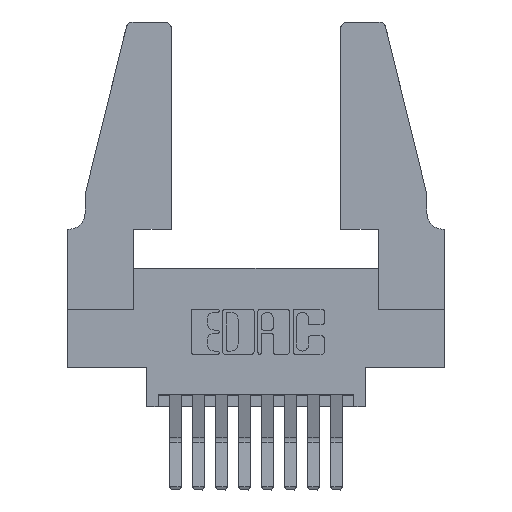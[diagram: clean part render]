
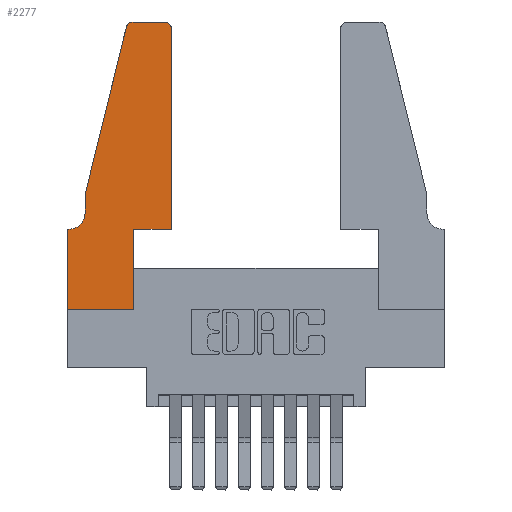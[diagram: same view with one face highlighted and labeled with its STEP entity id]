
A CAD part, top view. The second image highlights one B-rep face of the part: STEP entity #2277.
In plain terms, the highlighted planar face has unit normal (0, 0, 1).
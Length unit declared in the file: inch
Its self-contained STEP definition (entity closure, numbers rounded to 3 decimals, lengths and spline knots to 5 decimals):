
#139 = ORIENTED_EDGE ( 'NONE', *, *, #2441, .T. ) ;
#209 = CARTESIAN_POINT ( 'NONE',  ( 0.0755, 0.5, 0.37 ) ) ;
#359 = LINE ( 'NONE', #10617, #1563 ) ;
#665 = ORIENTED_EDGE ( 'NONE', *, *, #5520, .T. ) ;
#1165 = DIRECTION ( 'NONE',  ( 1., 0., 0. ) ) ;
#1204 = EDGE_CURVE ( 'NONE', #5422, #12656, #9728, .T. ) ;
#1392 = DIRECTION ( 'NONE',  ( -1., 0., 0. ) ) ;
#1563 = VECTOR ( 'NONE', #2473, 39.37008 ) ;
#1684 = DIRECTION ( 'NONE',  ( 0., -1., 0. ) ) ;
#1807 = VECTOR ( 'NONE', #3904, 39.37008 ) ;
#1826 = CARTESIAN_POINT ( 'NONE',  ( 0., 0., 0.37 ) ) ;
#2215 = VECTOR ( 'NONE', #1165, 39.37008 ) ;
#2277 = ADVANCED_FACE ( 'NONE', ( #2661 ), #8542, .T. ) ;
#2283 = VERTEX_POINT ( 'NONE', #11333 ) ;
#2441 = EDGE_CURVE ( 'NONE', #2283, #3994, #6580, .T. ) ;
#2448 = CIRCLE ( 'NONE', #3282, 0.03 ) ;
#2473 = DIRECTION ( 'NONE',  ( 0., 1., 0. ) ) ;
#2598 = CARTESIAN_POINT ( 'NONE',  ( 0.2865, 0.35, 0.37 ) ) ;
#2661 = FACE_OUTER_BOUND ( 'NONE', #2886, .T. ) ;
#2803 = LINE ( 'NONE', #9592, #13189 ) ;
#2817 = EDGE_CURVE ( 'NONE', #11545, #5595, #7525, .T. ) ;
#2837 = VERTEX_POINT ( 'NONE', #6873 ) ;
#2886 = EDGE_LOOP ( 'NONE', ( #139, #12139, #8908, #665, #12896, #9396, #6547, #11889, #8979, #6647, #8243, #10507 ) ) ;
#3049 = CARTESIAN_POINT ( 'NONE',  ( 0.0055, 0.35, 0.37 ) ) ;
#3071 = EDGE_CURVE ( 'NONE', #6088, #13042, #9677, .T. ) ;
#3072 = CARTESIAN_POINT ( 'NONE',  ( 0.4505, 0.35, 0.37 ) ) ;
#3123 = CARTESIAN_POINT ( 'NONE',  ( 0.4505, 0.35, 0.37 ) ) ;
#3135 = AXIS2_PLACEMENT_3D ( 'NONE', #8990, #8208, #11821 ) ;
#3225 = VERTEX_POINT ( 'NONE', #209 ) ;
#3266 = VECTOR ( 'NONE', #9991, 39.37008 ) ;
#3282 = AXIS2_PLACEMENT_3D ( 'NONE', #6283, #13174, #7293 ) ;
#3471 = EDGE_CURVE ( 'NONE', #12656, #11545, #2803, .T. ) ;
#3514 = VECTOR ( 'NONE', #6113, 39.37008 ) ;
#3708 = DIRECTION ( 'NONE',  ( 0., 0., -1. ) ) ;
#3747 = AXIS2_PLACEMENT_3D ( 'NONE', #7775, #3708, #11524 ) ;
#3904 = DIRECTION ( 'NONE',  ( 1., 0., 0. ) ) ;
#3994 = VERTEX_POINT ( 'NONE', #5449 ) ;
#4210 = EDGE_CURVE ( 'NONE', #3994, #2837, #5448, .T. ) ;
#4516 = VECTOR ( 'NONE', #7219, 39.37008 ) ;
#4773 = DIRECTION ( 'NONE',  ( 0., 0., 1. ) ) ;
#4895 = LINE ( 'NONE', #3123, #11602 ) ;
#5058 = LINE ( 'NONE', #5441, #2215 ) ;
#5085 = EDGE_CURVE ( 'NONE', #2837, #3225, #5741, .T. ) ;
#5121 = AXIS2_PLACEMENT_3D ( 'NONE', #10730, #4773, #11746 ) ;
#5422 = VERTEX_POINT ( 'NONE', #9725 ) ;
#5441 = CARTESIAN_POINT ( 'NONE',  ( 0., 0., 0.37 ) ) ;
#5448 = CIRCLE ( 'NONE', #5121, 0.03 ) ;
#5449 = CARTESIAN_POINT ( 'NONE',  ( 0.284, 1.25, 0.37 ) ) ;
#5520 = EDGE_CURVE ( 'NONE', #3225, #5422, #11314, .T. ) ;
#5595 = VERTEX_POINT ( 'NONE', #1826 ) ;
#5741 = LINE ( 'NONE', #8023, #3266 ) ;
#5845 = CARTESIAN_POINT ( 'NONE',  ( 0.4505, 0.35, 0.37 ) ) ;
#5930 = CARTESIAN_POINT ( 'NONE',  ( 0.4505, 1.22, 0.37 ) ) ;
#6038 = CARTESIAN_POINT ( 'NONE',  ( 0.2605, 1.25, 0.37 ) ) ;
#6088 = VERTEX_POINT ( 'NONE', #2598 ) ;
#6113 = DIRECTION ( 'NONE',  ( -1., 0., 0. ) ) ;
#6164 = VERTEX_POINT ( 'NONE', #5930 ) ;
#6283 = CARTESIAN_POINT ( 'NONE',  ( 0.4205, 1.22, 0.37 ) ) ;
#6367 = VERTEX_POINT ( 'NONE', #12958 ) ;
#6483 = EDGE_CURVE ( 'NONE', #13042, #6164, #4895, .T. ) ;
#6547 = ORIENTED_EDGE ( 'NONE', *, *, #2817, .T. ) ;
#6580 = LINE ( 'NONE', #6038, #3514 ) ;
#6608 = EDGE_CURVE ( 'NONE', #5595, #6367, #5058, .T. ) ;
#6647 = ORIENTED_EDGE ( 'NONE', *, *, #3071, .T. ) ;
#6873 = CARTESIAN_POINT ( 'NONE',  ( 0.25487, 1.22718, 0.37 ) ) ;
#7073 = CARTESIAN_POINT ( 'NONE',  ( 0., 0., 0.37 ) ) ;
#7219 = DIRECTION ( 'NONE',  ( 0., -1., 0. ) ) ;
#7293 = DIRECTION ( 'NONE',  ( 1., 0., 0. ) ) ;
#7525 = LINE ( 'NONE', #7073, #4516 ) ;
#7775 = CARTESIAN_POINT ( 'NONE',  ( 0.0055, 0.42, 0.37 ) ) ;
#8023 = CARTESIAN_POINT ( 'NONE',  ( 0.0755, 0.5, 0.37 ) ) ;
#8208 = DIRECTION ( 'NONE',  ( 0., 0., 1. ) ) ;
#8243 = ORIENTED_EDGE ( 'NONE', *, *, #6483, .T. ) ;
#8542 = PLANE ( 'NONE',  #3135 ) ;
#8908 = ORIENTED_EDGE ( 'NONE', *, *, #5085, .T. ) ;
#8919 = CARTESIAN_POINT ( 'NONE',  ( 0.0755, 0.5, 0.37 ) ) ;
#8979 = ORIENTED_EDGE ( 'NONE', *, *, #11957, .T. ) ;
#8990 = CARTESIAN_POINT ( 'NONE',  ( 0., 0.35, 0.37 ) ) ;
#9018 = CARTESIAN_POINT ( 'NONE',  ( 0., 0.35, 0.37 ) ) ;
#9396 = ORIENTED_EDGE ( 'NONE', *, *, #3471, .T. ) ;
#9592 = CARTESIAN_POINT ( 'NONE',  ( 0.0755, 0.35, 0.37 ) ) ;
#9677 = LINE ( 'NONE', #3072, #1807 ) ;
#9725 = CARTESIAN_POINT ( 'NONE',  ( 0.0755, 0.42, 0.37 ) ) ;
#9728 = CIRCLE ( 'NONE', #3747, 0.07 ) ;
#9991 = DIRECTION ( 'NONE',  ( -0.239, -0.971, 0. ) ) ;
#10350 = EDGE_CURVE ( 'NONE', #6164, #2283, #2448, .T. ) ;
#10507 = ORIENTED_EDGE ( 'NONE', *, *, #10350, .T. ) ;
#10617 = CARTESIAN_POINT ( 'NONE',  ( 0.2865, 0.35, 0.37 ) ) ;
#10730 = CARTESIAN_POINT ( 'NONE',  ( 0.284, 1.22, 0.37 ) ) ;
#11006 = VECTOR ( 'NONE', #1684, 39.37008 ) ;
#11218 = DIRECTION ( 'NONE',  ( 0., 1., 0. ) ) ;
#11314 = LINE ( 'NONE', #8919, #11006 ) ;
#11333 = CARTESIAN_POINT ( 'NONE',  ( 0.4205, 1.25, 0.37 ) ) ;
#11524 = DIRECTION ( 'NONE',  ( -1., 0., 0. ) ) ;
#11545 = VERTEX_POINT ( 'NONE', #9018 ) ;
#11602 = VECTOR ( 'NONE', #11218, 39.37008 ) ;
#11746 = DIRECTION ( 'NONE',  ( 1., 0., 0. ) ) ;
#11821 = DIRECTION ( 'NONE',  ( 1., 0., 0. ) ) ;
#11889 = ORIENTED_EDGE ( 'NONE', *, *, #6608, .T. ) ;
#11957 = EDGE_CURVE ( 'NONE', #6367, #6088, #359, .T. ) ;
#12139 = ORIENTED_EDGE ( 'NONE', *, *, #4210, .T. ) ;
#12656 = VERTEX_POINT ( 'NONE', #3049 ) ;
#12896 = ORIENTED_EDGE ( 'NONE', *, *, #1204, .T. ) ;
#12958 = CARTESIAN_POINT ( 'NONE',  ( 0.2865, 0., 0.37 ) ) ;
#13042 = VERTEX_POINT ( 'NONE', #5845 ) ;
#13174 = DIRECTION ( 'NONE',  ( 0., 0., 1. ) ) ;
#13189 = VECTOR ( 'NONE', #1392, 39.37008 ) ;
